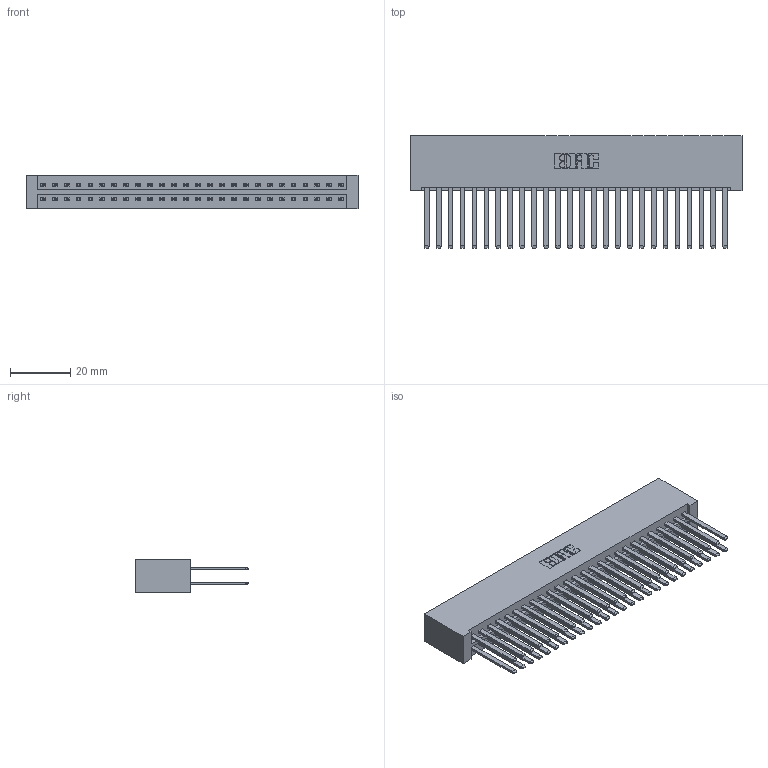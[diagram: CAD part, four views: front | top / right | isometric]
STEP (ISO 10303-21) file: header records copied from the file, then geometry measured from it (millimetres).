
FILE_DESCRIPTION (( 'STEP AP203' ), '1' );
FILE_NAME ('336-052-541-801.STEP', '2020-08-08T00:12:48', ( '' ), ( '' ), 'SwSTEP 2.0', 'SolidWorks 2020', '' );
FILE_SCHEMA (( 'CONFIG_CONTROL_DESIGN' ));
Length unit declared in the file: inch
Products named in the file (3): 336-052-541-801; 336-290-001_336-290-541; 336 Part_Lugless
Assembly tree (53 placements, depth 2):
  336-052-541-801
    336 Part_Lugless
    336-290-001_336-290-541  x52
Bounding box: 110.13 x 37.34 x 11.1 mm (x, y, z)
Volume: 18174.4 mm3; surface area: 23120.7 mm2
Topology: 53 solids, 53 shells, 2290 faces, 6891 edges, 4558 vertices
Faces by surface type: plane 1418, cylinder 872
Entity records: 21670 total; most frequent: CARTESIAN_POINT 3745, ORIENTED_EDGE 3582, DIRECTION 3111, EDGE_CURVE 1791, LINE 1667, VECTOR 1667, VERTEX_POINT 1192, AXIS2_PLACEMENT_3D 722
